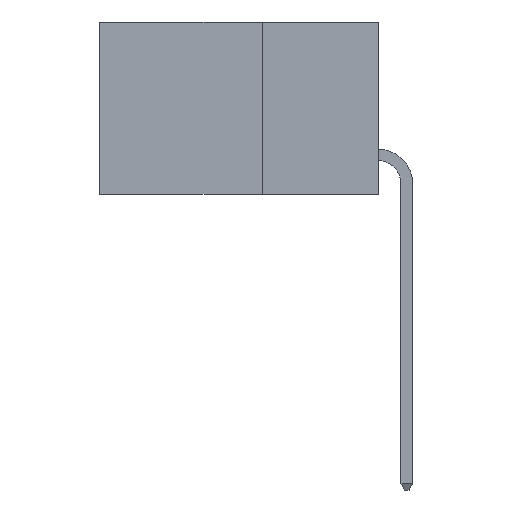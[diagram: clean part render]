
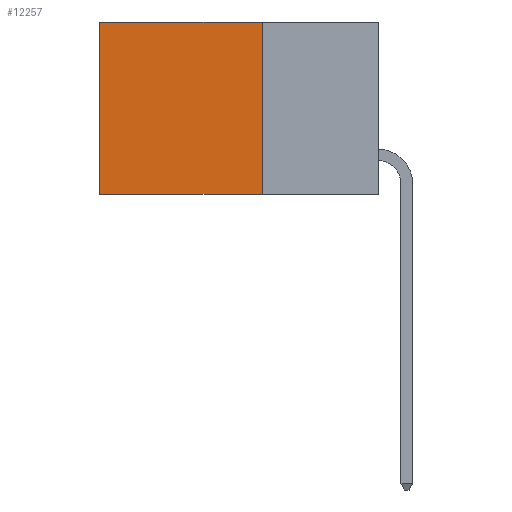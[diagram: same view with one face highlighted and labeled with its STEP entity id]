
A CAD part, left-side view. The second image highlights one B-rep face of the part: STEP entity #12257.
In plain terms, the highlighted planar face has unit normal (-1, 0, 0).
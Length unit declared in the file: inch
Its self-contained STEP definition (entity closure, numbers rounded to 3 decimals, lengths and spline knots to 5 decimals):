
#283 = VERTEX_POINT ( 'NONE', #16518 ) ;
#671 = VERTEX_POINT ( 'NONE', #5690 ) ;
#1839 = EDGE_CURVE ( 'NONE', #18393, #671, #9782, .T. ) ;
#2853 = CARTESIAN_POINT ( 'NONE',  ( 0.2615, 0.6, -0.37 ) ) ;
#3535 = LINE ( 'NONE', #2853, #7514 ) ;
#3626 = VERTEX_POINT ( 'NONE', #18668 ) ;
#4802 = ORIENTED_EDGE ( 'NONE', *, *, #16890, .T. ) ;
#5655 = VECTOR ( 'NONE', #10960, 39.37008 ) ;
#5690 = CARTESIAN_POINT ( 'NONE',  ( 0.2615, 0.6, 0. ) ) ;
#6858 = FACE_OUTER_BOUND ( 'NONE', #9411, .T. ) ;
#7514 = VECTOR ( 'NONE', #9599, 39.37008 ) ;
#8208 = DIRECTION ( 'NONE',  ( 0., 0., -1. ) ) ;
#8218 = AXIS2_PLACEMENT_3D ( 'NONE', #8706, #8337, #8208 ) ;
#8337 = DIRECTION ( 'NONE',  ( 1., 0., 0. ) ) ;
#8519 = PLANE ( 'NONE',  #8218 ) ;
#8706 = CARTESIAN_POINT ( 'NONE',  ( 0.2615, 0.25, -0.37 ) ) ;
#9411 = EDGE_LOOP ( 'NONE', ( #4802, #15882, #11362, #10490 ) ) ;
#9599 = DIRECTION ( 'NONE',  ( 0., 0., -1. ) ) ;
#9782 = LINE ( 'NONE', #11077, #17967 ) ;
#10031 = DIRECTION ( 'NONE',  ( 0., 1., 0. ) ) ;
#10490 = ORIENTED_EDGE ( 'NONE', *, *, #1839, .T. ) ;
#10688 = LINE ( 'NONE', #19109, #5655 ) ;
#10960 = DIRECTION ( 'NONE',  ( 0., 0., -1. ) ) ;
#11077 = CARTESIAN_POINT ( 'NONE',  ( 0.2615, 0.25, 0. ) ) ;
#11362 = ORIENTED_EDGE ( 'NONE', *, *, #15945, .F. ) ;
#11850 = CARTESIAN_POINT ( 'NONE',  ( 0.2615, 0.25, 0. ) ) ;
#12257 = ADVANCED_FACE ( 'NONE', ( #6858 ), #8519, .F. ) ;
#14390 = DIRECTION ( 'NONE',  ( 0., 1., 0. ) ) ;
#14691 = EDGE_CURVE ( 'NONE', #283, #3626, #18409, .T. ) ;
#15882 = ORIENTED_EDGE ( 'NONE', *, *, #14691, .F. ) ;
#15945 = EDGE_CURVE ( 'NONE', #18393, #283, #10688, .T. ) ;
#16028 = CARTESIAN_POINT ( 'NONE',  ( 0.2615, 0.25, -0.37 ) ) ;
#16518 = CARTESIAN_POINT ( 'NONE',  ( 0.2615, 0.25, -0.37 ) ) ;
#16890 = EDGE_CURVE ( 'NONE', #671, #3626, #3535, .T. ) ;
#17880 = VECTOR ( 'NONE', #14390, 39.37008 ) ;
#17967 = VECTOR ( 'NONE', #10031, 39.37008 ) ;
#18393 = VERTEX_POINT ( 'NONE', #11850 ) ;
#18409 = LINE ( 'NONE', #16028, #17880 ) ;
#18668 = CARTESIAN_POINT ( 'NONE',  ( 0.2615, 0.6, -0.37 ) ) ;
#19109 = CARTESIAN_POINT ( 'NONE',  ( 0.2615, 0.25, -0.37 ) ) ;
